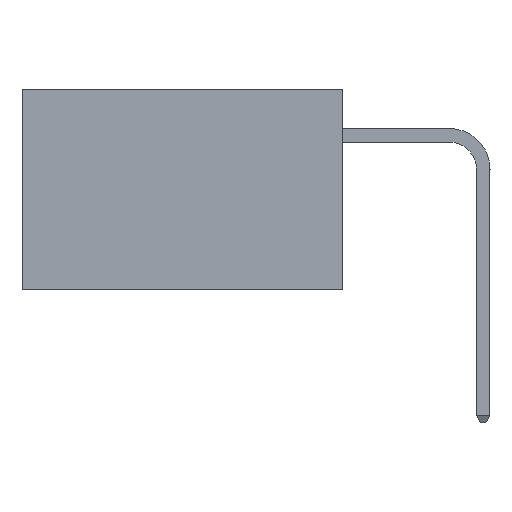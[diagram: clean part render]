
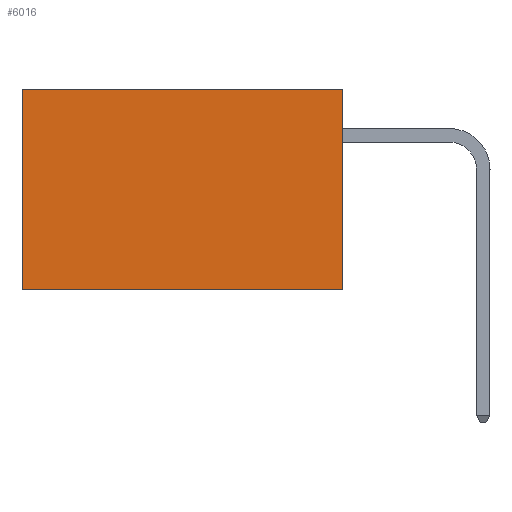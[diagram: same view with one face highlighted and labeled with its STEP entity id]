
A CAD part, left-side view. The second image highlights one B-rep face of the part: STEP entity #6016.
In plain terms, the highlighted planar face has unit normal (-1, 0, 0).
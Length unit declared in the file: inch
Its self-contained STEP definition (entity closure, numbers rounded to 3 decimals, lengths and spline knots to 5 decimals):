
#1271 = DIRECTION ( 'NONE',  ( 0., 0., -1. ) ) ;
#1293 = DIRECTION ( 'NONE',  ( 1., 0., 0. ) ) ;
#1446 = PLANE ( 'NONE',  #20253 ) ;
#1723 = CARTESIAN_POINT ( 'NONE',  ( 0.277, 0., -0.37 ) ) ;
#4925 = ORIENTED_EDGE ( 'NONE', *, *, #14839, .T. ) ;
#5834 = EDGE_CURVE ( 'NONE', #22678, #10986, #23650, .T. ) ;
#6016 = ADVANCED_FACE ( 'NONE', ( #19396 ), #1446, .F. ) ;
#7746 = DIRECTION ( 'NONE',  ( 0., 1., 0. ) ) ;
#9043 = ORIENTED_EDGE ( 'NONE', *, *, #5834, .F. ) ;
#9503 = CARTESIAN_POINT ( 'NONE',  ( 0.277, 0., -0.37 ) ) ;
#9606 = VERTEX_POINT ( 'NONE', #14089 ) ;
#10272 = CARTESIAN_POINT ( 'NONE',  ( 0.277, 0.59, -0.37 ) ) ;
#10986 = VERTEX_POINT ( 'NONE', #15238 ) ;
#12881 = EDGE_CURVE ( 'NONE', #9606, #15324, #20744, .T. ) ;
#13575 = VECTOR ( 'NONE', #22905, 39.37008 ) ;
#14089 = CARTESIAN_POINT ( 'NONE',  ( 0.277, 0., 0. ) ) ;
#14839 = EDGE_CURVE ( 'NONE', #15324, #10986, #22409, .T. ) ;
#15238 = CARTESIAN_POINT ( 'NONE',  ( 0.277, 0.59, -0.37 ) ) ;
#15324 = VERTEX_POINT ( 'NONE', #25331 ) ;
#15478 = ORIENTED_EDGE ( 'NONE', *, *, #21943, .F. ) ;
#17043 = CARTESIAN_POINT ( 'NONE',  ( 0.277, 0., -0.37 ) ) ;
#17094 = CARTESIAN_POINT ( 'NONE',  ( 0.277, 0., -0.37 ) ) ;
#17244 = VECTOR ( 'NONE', #23951, 39.37008 ) ;
#18298 = DIRECTION ( 'NONE',  ( 0., 1., 0. ) ) ;
#18373 = CARTESIAN_POINT ( 'NONE',  ( 0.277, 0., 0. ) ) ;
#18801 = LINE ( 'NONE', #17043, #13575 ) ;
#19396 = FACE_OUTER_BOUND ( 'NONE', #21282, .T. ) ;
#20114 = VECTOR ( 'NONE', #18298, 39.37008 ) ;
#20253 = AXIS2_PLACEMENT_3D ( 'NONE', #1723, #1293, #1271 ) ;
#20744 = LINE ( 'NONE', #18373, #20114 ) ;
#21282 = EDGE_LOOP ( 'NONE', ( #4925, #9043, #15478, #22969 ) ) ;
#21943 = EDGE_CURVE ( 'NONE', #9606, #22678, #18801, .T. ) ;
#22409 = LINE ( 'NONE', #10272, #17244 ) ;
#22678 = VERTEX_POINT ( 'NONE', #17094 ) ;
#22905 = DIRECTION ( 'NONE',  ( 0., 0., -1. ) ) ;
#22969 = ORIENTED_EDGE ( 'NONE', *, *, #12881, .T. ) ;
#23055 = VECTOR ( 'NONE', #7746, 39.37008 ) ;
#23650 = LINE ( 'NONE', #9503, #23055 ) ;
#23951 = DIRECTION ( 'NONE',  ( 0., 0., -1. ) ) ;
#25331 = CARTESIAN_POINT ( 'NONE',  ( 0.277, 0.59, 0. ) ) ;
